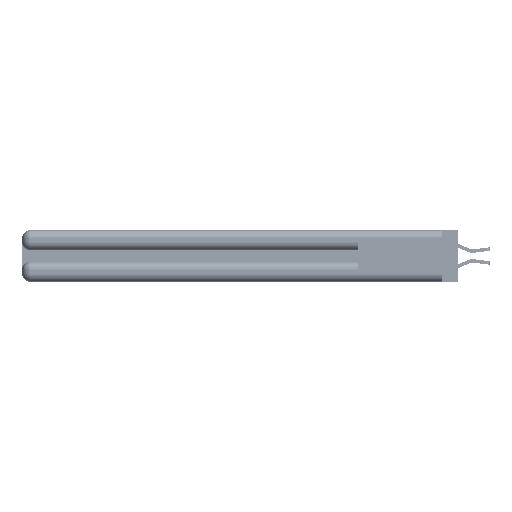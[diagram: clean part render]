
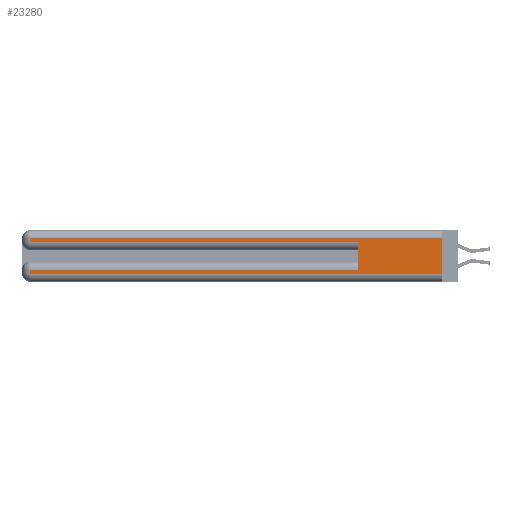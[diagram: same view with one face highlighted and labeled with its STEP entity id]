
A CAD part, left-side view. The second image highlights one B-rep face of the part: STEP entity #23280.
In plain terms, the highlighted planar face has unit normal (-1, 0, 0).
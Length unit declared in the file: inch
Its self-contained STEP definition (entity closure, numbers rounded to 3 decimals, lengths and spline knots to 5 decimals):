
#284 = EDGE_CURVE ( 'NONE', #25512, #9177, #11407, .T. ) ;
#616 = DIRECTION ( 'NONE',  ( 0., 0., 1. ) ) ;
#2034 = DIRECTION ( 'NONE',  ( 0., 0., -1. ) ) ;
#3941 = EDGE_CURVE ( 'NONE', #16160, #27918, #17414, .T. ) ;
#5650 = VECTOR ( 'NONE', #24379, 39.37008 ) ;
#5854 = CARTESIAN_POINT ( 'NONE',  ( 0., 2.94, 0.37 ) ) ;
#6561 = CARTESIAN_POINT ( 'NONE',  ( 0., 0.6, 0.085 ) ) ;
#7117 = LINE ( 'NONE', #32452, #33170 ) ;
#7898 = LINE ( 'NONE', #20061, #33935 ) ;
#8552 = DIRECTION ( 'NONE',  ( 0., -1., 0. ) ) ;
#9177 = VERTEX_POINT ( 'NONE', #9318 ) ;
#9185 = CARTESIAN_POINT ( 'NONE',  ( 0., 0., 0.06 ) ) ;
#9318 = CARTESIAN_POINT ( 'NONE',  ( 0., 0., 0.06 ) ) ;
#9644 = EDGE_CURVE ( 'NONE', #37121, #16160, #35767, .T. ) ;
#9708 = CARTESIAN_POINT ( 'NONE',  ( 0., 2.94, 0.285 ) ) ;
#9741 = EDGE_CURVE ( 'NONE', #34496, #21661, #7117, .T. ) ;
#10014 = VECTOR ( 'NONE', #43267, 39.37008 ) ;
#10563 = VERTEX_POINT ( 'NONE', #41204 ) ;
#10715 = CARTESIAN_POINT ( 'NONE',  ( 0., 0., 0.37 ) ) ;
#10855 = DIRECTION ( 'NONE',  ( 0., 0., -1. ) ) ;
#11310 = DIRECTION ( 'NONE',  ( 1., 0., 0. ) ) ;
#11407 = LINE ( 'NONE', #10715, #5650 ) ;
#11648 = CARTESIAN_POINT ( 'NONE',  ( 0., 2.94, 0.06 ) ) ;
#12287 = ORIENTED_EDGE ( 'NONE', *, *, #19441, .T. ) ;
#13941 = EDGE_LOOP ( 'NONE', ( #16988, #17712, #12287, #39747, #38812, #16810, #36883, #16979 ) ) ;
#14008 = VECTOR ( 'NONE', #2034, 39.37008 ) ;
#14793 = CARTESIAN_POINT ( 'NONE',  ( 0., 0., 0.085 ) ) ;
#14889 = AXIS2_PLACEMENT_3D ( 'NONE', #17970, #11310, #10855 ) ;
#15203 = EDGE_CURVE ( 'NONE', #37121, #21661, #7898, .T. ) ;
#15296 = EDGE_CURVE ( 'NONE', #25512, #10563, #23354, .T. ) ;
#16160 = VERTEX_POINT ( 'NONE', #30843 ) ;
#16320 = FACE_OUTER_BOUND ( 'NONE', #13941, .T. ) ;
#16810 = ORIENTED_EDGE ( 'NONE', *, *, #9644, .T. ) ;
#16979 = ORIENTED_EDGE ( 'NONE', *, *, #41471, .T. ) ;
#16988 = ORIENTED_EDGE ( 'NONE', *, *, #284, .F. ) ;
#17414 = LINE ( 'NONE', #24949, #18478 ) ;
#17712 = ORIENTED_EDGE ( 'NONE', *, *, #15296, .T. ) ;
#17970 = CARTESIAN_POINT ( 'NONE',  ( 0., 0., 0.37 ) ) ;
#18478 = VECTOR ( 'NONE', #25099, 39.37008 ) ;
#19441 = EDGE_CURVE ( 'NONE', #10563, #34496, #32645, .T. ) ;
#20061 = CARTESIAN_POINT ( 'NONE',  ( 0., 0.6, 0.145 ) ) ;
#21255 = PLANE ( 'NONE',  #14889 ) ;
#21661 = VERTEX_POINT ( 'NONE', #31742 ) ;
#23280 = ADVANCED_FACE ( 'NONE', ( #16320 ), #21255, .F. ) ;
#23354 = LINE ( 'NONE', #31836, #42936 ) ;
#24379 = DIRECTION ( 'NONE',  ( 0., 0., -1. ) ) ;
#24949 = CARTESIAN_POINT ( 'NONE',  ( 0., 2.94, 0.37 ) ) ;
#25099 = DIRECTION ( 'NONE',  ( 0., 0., -1. ) ) ;
#25512 = VERTEX_POINT ( 'NONE', #33877 ) ;
#27918 = VERTEX_POINT ( 'NONE', #11648 ) ;
#30843 = CARTESIAN_POINT ( 'NONE',  ( 0., 2.94, 0.085 ) ) ;
#31577 = DIRECTION ( 'NONE',  ( 0., 1., 0. ) ) ;
#31742 = CARTESIAN_POINT ( 'NONE',  ( 0., 0.6, 0.285 ) ) ;
#31836 = CARTESIAN_POINT ( 'NONE',  ( 0., 0., 0.31 ) ) ;
#31992 = DIRECTION ( 'NONE',  ( 0., 1., 0. ) ) ;
#32452 = CARTESIAN_POINT ( 'NONE',  ( 0., 0., 0.285 ) ) ;
#32645 = LINE ( 'NONE', #5854, #14008 ) ;
#33162 = VECTOR ( 'NONE', #31577, 39.37008 ) ;
#33170 = VECTOR ( 'NONE', #8552, 39.37008 ) ;
#33877 = CARTESIAN_POINT ( 'NONE',  ( 0., 0., 0.31 ) ) ;
#33935 = VECTOR ( 'NONE', #616, 39.37008 ) ;
#34496 = VERTEX_POINT ( 'NONE', #9708 ) ;
#35767 = LINE ( 'NONE', #14793, #33162 ) ;
#36883 = ORIENTED_EDGE ( 'NONE', *, *, #3941, .T. ) ;
#37121 = VERTEX_POINT ( 'NONE', #6561 ) ;
#38812 = ORIENTED_EDGE ( 'NONE', *, *, #15203, .F. ) ;
#39747 = ORIENTED_EDGE ( 'NONE', *, *, #9741, .T. ) ;
#40251 = LINE ( 'NONE', #9185, #10014 ) ;
#41204 = CARTESIAN_POINT ( 'NONE',  ( 0., 2.94, 0.31 ) ) ;
#41471 = EDGE_CURVE ( 'NONE', #27918, #9177, #40251, .T. ) ;
#42936 = VECTOR ( 'NONE', #31992, 39.37008 ) ;
#43267 = DIRECTION ( 'NONE',  ( 0., -1., 0. ) ) ;
